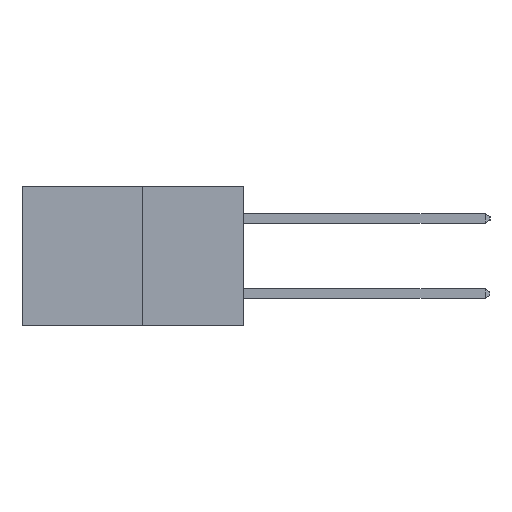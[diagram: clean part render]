
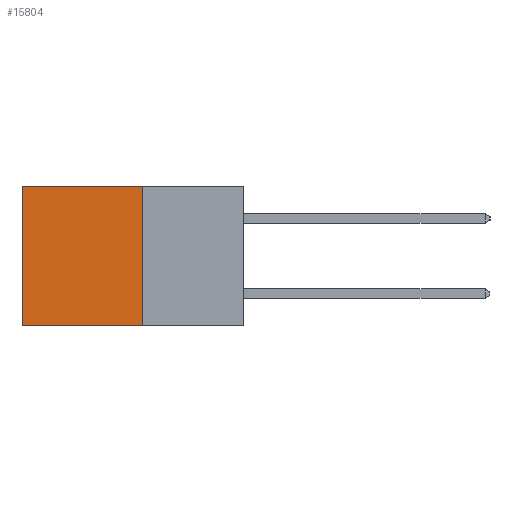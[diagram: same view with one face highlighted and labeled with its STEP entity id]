
A CAD part, left-side view. The second image highlights one B-rep face of the part: STEP entity #15804.
In plain terms, the highlighted planar face has unit normal (-1, 0, 0).
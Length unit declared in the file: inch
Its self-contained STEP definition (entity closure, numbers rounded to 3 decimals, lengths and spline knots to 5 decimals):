
#609 = VECTOR ( 'NONE', #1747, 39.37008 ) ;
#670 = EDGE_CURVE ( 'NONE', #16636, #17711, #3865, .T. ) ;
#691 = EDGE_CURVE ( 'NONE', #14543, #3731, #3598, .T. ) ;
#1747 = DIRECTION ( 'NONE',  ( 0., 1., 0. ) ) ;
#2196 = CARTESIAN_POINT ( 'NONE',  ( 0.277, 0.59, -0.37 ) ) ;
#2312 = EDGE_LOOP ( 'NONE', ( #17372, #7116, #12262, #4195 ) ) ;
#2410 = DIRECTION ( 'NONE',  ( 0., 0., -1. ) ) ;
#2474 = DIRECTION ( 'NONE',  ( 0., 0., -1. ) ) ;
#2743 = CARTESIAN_POINT ( 'NONE',  ( 0.277, 0.27, -0.37 ) ) ;
#3305 = PLANE ( 'NONE',  #10027 ) ;
#3407 = VECTOR ( 'NONE', #2474, 39.37008 ) ;
#3598 = LINE ( 'NONE', #7138, #18060 ) ;
#3731 = VERTEX_POINT ( 'NONE', #11537 ) ;
#3865 = LINE ( 'NONE', #7268, #3407 ) ;
#4195 = ORIENTED_EDGE ( 'NONE', *, *, #13661, .T. ) ;
#4405 = LINE ( 'NONE', #8928, #609 ) ;
#4758 = DIRECTION ( 'NONE',  ( 1., 0., 0. ) ) ;
#5378 = CARTESIAN_POINT ( 'NONE',  ( 0.277, 0.59, 0. ) ) ;
#7116 = ORIENTED_EDGE ( 'NONE', *, *, #9960, .F. ) ;
#7138 = CARTESIAN_POINT ( 'NONE',  ( 0.277, 0.27, -0.37 ) ) ;
#7268 = CARTESIAN_POINT ( 'NONE',  ( 0.277, 0.59, -0.37 ) ) ;
#8928 = CARTESIAN_POINT ( 'NONE',  ( 0.277, 0.27, 0. ) ) ;
#9960 = EDGE_CURVE ( 'NONE', #3731, #17711, #15691, .T. ) ;
#10027 = AXIS2_PLACEMENT_3D ( 'NONE', #13299, #4758, #14662 ) ;
#10744 = CARTESIAN_POINT ( 'NONE',  ( 0.277, 0.27, 0. ) ) ;
#11537 = CARTESIAN_POINT ( 'NONE',  ( 0.277, 0.27, -0.37 ) ) ;
#12031 = VECTOR ( 'NONE', #17209, 39.37008 ) ;
#12262 = ORIENTED_EDGE ( 'NONE', *, *, #691, .F. ) ;
#13245 = FACE_OUTER_BOUND ( 'NONE', #2312, .T. ) ;
#13299 = CARTESIAN_POINT ( 'NONE',  ( 0.277, 0.27, -0.37 ) ) ;
#13661 = EDGE_CURVE ( 'NONE', #14543, #16636, #4405, .T. ) ;
#14543 = VERTEX_POINT ( 'NONE', #10744 ) ;
#14662 = DIRECTION ( 'NONE',  ( 0., 0., -1. ) ) ;
#15691 = LINE ( 'NONE', #2743, #12031 ) ;
#15804 = ADVANCED_FACE ( 'NONE', ( #13245 ), #3305, .F. ) ;
#16636 = VERTEX_POINT ( 'NONE', #5378 ) ;
#17209 = DIRECTION ( 'NONE',  ( 0., 1., 0. ) ) ;
#17372 = ORIENTED_EDGE ( 'NONE', *, *, #670, .T. ) ;
#17711 = VERTEX_POINT ( 'NONE', #2196 ) ;
#18060 = VECTOR ( 'NONE', #2410, 39.37008 ) ;
